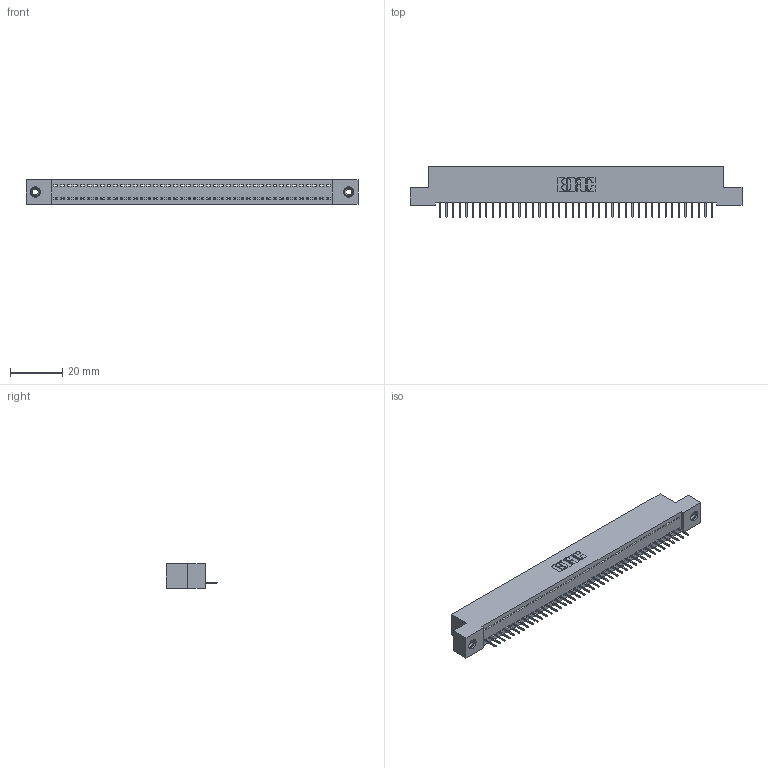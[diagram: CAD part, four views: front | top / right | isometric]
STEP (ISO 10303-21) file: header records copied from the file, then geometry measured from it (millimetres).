
FILE_DESCRIPTION (( 'STEP AP203' ), '1' );
FILE_NAME ('392-042-524-108.STEP', '2018-08-16T13:27:02', ( '' ), ( '' ), 'SwSTEP 2.0', 'SolidWorks 2016', '' );
FILE_SCHEMA (( 'CONFIG_CONTROL_DESIGN' ));
Length unit declared in the file: inch
Products named in the file (4): 342 Part_TI; 345-292-001_345-293-124; 345-250-001_345-250-003-102; 392-042-524-108
Assembly tree (45 placements, depth 2):
  392-042-524-108
    342 Part_TI
    345-292-001_345-293-124  x42
    345-250-001_345-250-003-102  x2
Bounding box: 127 x 19.69 x 9.4 mm (x, y, z)
Volume: 10963.8 mm3; surface area: 15602.3 mm2
Topology: 45 solids, 45 shells, 2774 faces, 7995 edges, 5154 vertices
Faces by surface type: plane 2114, cylinder 644, cone 12, torus 4
Entity records: 26804 total; most frequent: CARTESIAN_POINT 4603, ORIENTED_EDGE 4574, DIRECTION 3917, EDGE_CURVE 2287, LINE 2143, VECTOR 2143, VERTEX_POINT 1516, AXIS2_PLACEMENT_3D 887
